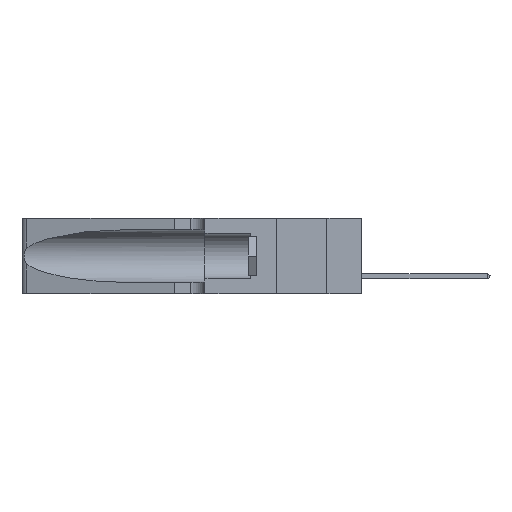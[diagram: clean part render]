
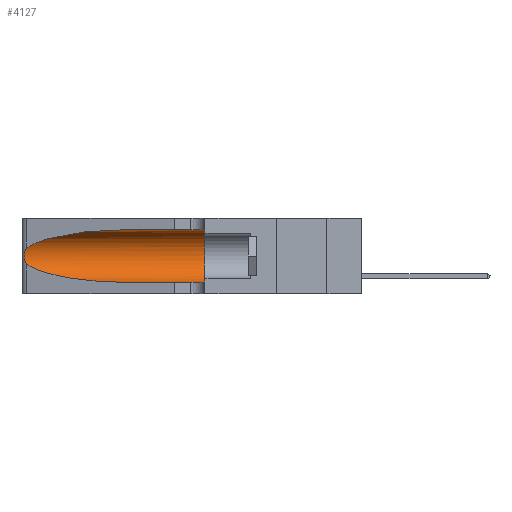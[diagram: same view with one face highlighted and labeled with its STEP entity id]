
A CAD part, left-side view. The second image highlights one B-rep face of the part: STEP entity #4127.
In plain terms, the highlighted cylindrical face has radius 3.308 mm (diameter 6.617 mm), a partial arc.
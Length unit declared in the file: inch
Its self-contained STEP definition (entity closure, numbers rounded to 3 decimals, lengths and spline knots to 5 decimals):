
#73 = VERTEX_POINT ( 'NONE', #23224 ) ;
#101 = CARTESIAN_POINT ( 'NONE',  ( 0.1305, 1.61858, 0.31525 ) ) ;
#203 = ORIENTED_EDGE ( 'NONE', *, *, #6644, .T. ) ;
#362 = AXIS2_PLACEMENT_3D ( 'NONE', #19050, #6513, #2310 ) ;
#700 = DIRECTION ( 'NONE',  ( 0., 0., 1. ) ) ;
#978 = AXIS2_PLACEMENT_3D ( 'NONE', #13477, #9151, #700 ) ;
#1409 = EDGE_CURVE ( 'NONE', #23331, #12118, #18061, .T. ) ;
#1876 = CARTESIAN_POINT ( 'NONE',  ( 0.26018, 1.23835, 0.19895 ) ) ;
#1944 = CARTESIAN_POINT ( 'NONE',  ( 0.25487, 1.22718, 0.22369 ) ) ;
#2310 = DIRECTION ( 'NONE',  ( 0., 0., -1. ) ) ;
#2666 = CARTESIAN_POINT ( 'NONE',  ( 0.25555, 1.22993, 0.14849 ) ) ;
#3684 = CARTESIAN_POINT ( 'NONE',  ( 0.25854, 1.2359, 0.20912 ) ) ;
#4127 = ADVANCED_FACE ( 'NONE', ( #13717 ), #6200, .F. ) ;
#4164 = ORIENTED_EDGE ( 'NONE', *, *, #25603, .F. ) ;
#4336 = VERTEX_POINT ( 'NONE', #24420 ) ;
#4804 = CARTESIAN_POINT ( 'NONE',  ( 0.2373, 1.15595, 0.08982 ) ) ;
#5880 = CARTESIAN_POINT ( 'NONE',  ( 0.25639, 1.23184, 0.21858 ) ) ;
#6200 = CYLINDRICAL_SURFACE ( 'NONE', #362, 0.13025 ) ;
#6513 = DIRECTION ( 'NONE',  ( 0., -1., 0. ) ) ;
#6644 = EDGE_CURVE ( 'NONE', #73, #13550, #22024, .T. ) ;
#6793 = CARTESIAN_POINT ( 'NONE',  ( 0.25487, 1.22718, 0.22369 ) ) ;
#6914 = CARTESIAN_POINT ( 'NONE',  ( 0.1305, 0.72297, 0.05475 ) ) ;
#7829 = CARTESIAN_POINT ( 'NONE',  ( 0.25787, 1.23484, 0.2124 ) ) ;
#8042 = EDGE_CURVE ( 'NONE', #13550, #4336, #23981, .T. ) ;
#8180 = CARTESIAN_POINT ( 'NONE',  ( 0.1305, 0.35, 0.05475 ) ) ;
#9151 = DIRECTION ( 'NONE',  ( 0., 1., 0. ) ) ;
#9198 = CARTESIAN_POINT ( 'NONE',  ( 0.1305, 0.72297, 0.05475 ) ) ;
#10470 = CIRCLE ( 'NONE', #978, 0.13025 ) ;
#11084 = CARTESIAN_POINT ( 'NONE',  ( 0.25487, 1.22718, 0.14631 ) ) ;
#12118 = VERTEX_POINT ( 'NONE', #8180 ) ;
#12304 = CARTESIAN_POINT ( 'NONE',  ( 0.1305, 0.72297, 0.31525 ) ) ;
#12448 = ORIENTED_EDGE ( 'NONE', *, *, #1409, .T. ) ;
#12487 = CARTESIAN_POINT ( 'NONE',  ( 0.18966, 0.96281, 0.31525 ) ) ;
#13458 = CARTESIAN_POINT ( 'NONE',  ( 0.1305, 0.35, 0.31525 ) ) ;
#13477 = CARTESIAN_POINT ( 'NONE',  ( 0.1305, 0.35, 0.185 ) ) ;
#13550 = VERTEX_POINT ( 'NONE', #6793 ) ;
#13717 = FACE_OUTER_BOUND ( 'NONE', #26006, .T. ) ;
#13735 =( BOUNDED_CURVE ( )  B_SPLINE_CURVE ( 3, ( #17434, #4804, #19552, #6914 ),
 .UNSPECIFIED., .F., .F. ) 
 B_SPLINE_CURVE_WITH_KNOTS ( ( 4, 4 ),
 ( 3.44316, 4.71239 ),
 .UNSPECIFIED. ) 
 CURVE ( )  GEOMETRIC_REPRESENTATION_ITEM ( )  RATIONAL_B_SPLINE_CURVE ( ( 1., 0.87, 0.87, 1. ) ) 
 REPRESENTATION_ITEM ( '' )  );
#13738 = ORIENTED_EDGE ( 'NONE', *, *, #17093, .F. ) ;
#14260 = CARTESIAN_POINT ( 'NONE',  ( 0.26017, 1.23833, 0.17102 ) ) ;
#14435 = CARTESIAN_POINT ( 'NONE',  ( 0.25555, 1.22994, 0.2215 ) ) ;
#14589 = CARTESIAN_POINT ( 'NONE',  ( 0.2373, 1.15595, 0.28018 ) ) ;
#15181 = VECTOR ( 'NONE', #20821, 39.37008 ) ;
#16560 = CARTESIAN_POINT ( 'NONE',  ( 0.26075, 1.23896, 0.178 ) ) ;
#17093 = EDGE_CURVE ( 'NONE', #25202, #12118, #10470, .T. ) ;
#17434 = CARTESIAN_POINT ( 'NONE',  ( 0.25487, 1.22718, 0.14631 ) ) ;
#18061 = LINE ( 'NONE', #21136, #26153 ) ;
#18096 = EDGE_CURVE ( 'NONE', #4336, #23331, #13735, .T. ) ;
#19050 = CARTESIAN_POINT ( 'NONE',  ( 0.1305, 1.61858, 0.185 ) ) ;
#19552 = CARTESIAN_POINT ( 'NONE',  ( 0.18966, 0.96281, 0.05475 ) ) ;
#19599 = CARTESIAN_POINT ( 'NONE',  ( 0.25639, 1.23186, 0.15144 ) ) ;
#20074 = ORIENTED_EDGE ( 'NONE', *, *, #8042, .T. ) ;
#20150 = LINE ( 'NONE', #101, #15181 ) ;
#20821 = DIRECTION ( 'NONE',  ( 0., -1., 0. ) ) ;
#21136 = CARTESIAN_POINT ( 'NONE',  ( 0.1305, 1.61858, 0.05475 ) ) ;
#22024 =( BOUNDED_CURVE ( )  B_SPLINE_CURVE ( 3, ( #12304, #12487, #14589, #1944 ),
 .UNSPECIFIED., .F., .T. ) 
 B_SPLINE_CURVE_WITH_KNOTS ( ( 4, 4 ),
 ( 1.5708, 2.84003 ),
 .UNSPECIFIED. ) 
 CURVE ( )  GEOMETRIC_REPRESENTATION_ITEM ( )  RATIONAL_B_SPLINE_CURVE ( ( 1., 0.87, 0.87, 1. ) ) 
 REPRESENTATION_ITEM ( '' )  );
#22555 = CARTESIAN_POINT ( 'NONE',  ( 0.26075, 1.23896, 0.19203 ) ) ;
#23224 = CARTESIAN_POINT ( 'NONE',  ( 0.1305, 0.72297, 0.31525 ) ) ;
#23331 = VERTEX_POINT ( 'NONE', #9198 ) ;
#23981 = B_SPLINE_CURVE_WITH_KNOTS ( 'NONE', 3,
 ( #24777, #14435, #5880, #7829, #3684, #1876, #22555, #16560, #14260, #27016, #26658, #19599, #2666, #11084 ),
 .UNSPECIFIED., .F., .F.,
 ( 4, 2, 2, 2, 2, 2, 4 ),
 ( 0., 0.00027, 0.00053, 0.00107, 0.0016, 0.00187, 0.00214 ),
 .UNSPECIFIED. ) ;
#24420 = CARTESIAN_POINT ( 'NONE',  ( 0.25487, 1.22718, 0.14631 ) ) ;
#24777 = CARTESIAN_POINT ( 'NONE',  ( 0.25487, 1.22718, 0.22369 ) ) ;
#25202 = VERTEX_POINT ( 'NONE', #13458 ) ;
#25203 = DIRECTION ( 'NONE',  ( 0., -1., 0. ) ) ;
#25603 = EDGE_CURVE ( 'NONE', #73, #25202, #20150, .T. ) ;
#26006 = EDGE_LOOP ( 'NONE', ( #203, #20074, #26128, #12448, #13738, #4164 ) ) ;
#26128 = ORIENTED_EDGE ( 'NONE', *, *, #18096, .T. ) ;
#26153 = VECTOR ( 'NONE', #25203, 39.37008 ) ;
#26658 = CARTESIAN_POINT ( 'NONE',  ( 0.25789, 1.23486, 0.15765 ) ) ;
#27016 = CARTESIAN_POINT ( 'NONE',  ( 0.25856, 1.23593, 0.16098 ) ) ;
